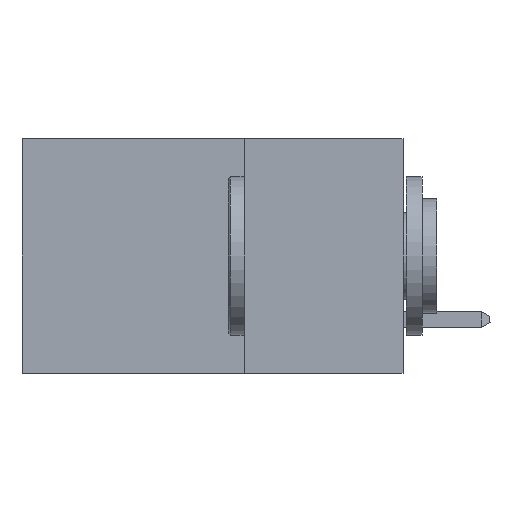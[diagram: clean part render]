
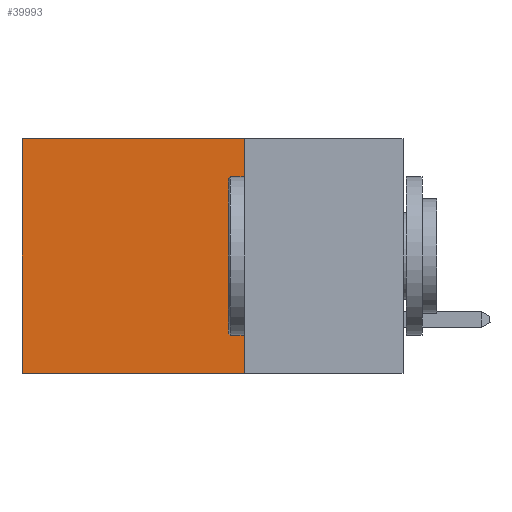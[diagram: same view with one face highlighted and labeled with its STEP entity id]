
A CAD part, left-side view. The second image highlights one B-rep face of the part: STEP entity #39993.
In plain terms, the highlighted planar face has unit normal (-1, 0, 0).
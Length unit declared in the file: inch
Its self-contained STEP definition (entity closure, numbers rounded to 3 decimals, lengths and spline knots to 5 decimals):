
#28 = EDGE_CURVE ( 'NONE', #30803, #10720, #9996, .T. ) ;
#980 = FACE_OUTER_BOUND ( 'NONE', #20535, .T. ) ;
#2550 = CARTESIAN_POINT ( 'NONE',  ( 0.2875, 0.25, 0. ) ) ;
#3827 = PLANE ( 'NONE',  #40299 ) ;
#6560 = DIRECTION ( 'NONE',  ( 0., 0., -1. ) ) ;
#7471 = ORIENTED_EDGE ( 'NONE', *, *, #28, .T. ) ;
#7860 = EDGE_CURVE ( 'NONE', #35607, #10720, #25566, .T. ) ;
#9996 = LINE ( 'NONE', #38169, #14913 ) ;
#10720 = VERTEX_POINT ( 'NONE', #34010 ) ;
#11876 = CARTESIAN_POINT ( 'NONE',  ( 0.2875, 0.25, 0. ) ) ;
#14913 = VECTOR ( 'NONE', #19667, 39.37008 ) ;
#15491 = VECTOR ( 'NONE', #36785, 39.37008 ) ;
#16440 = LINE ( 'NONE', #11876, #15491 ) ;
#17314 = VECTOR ( 'NONE', #28968, 39.37008 ) ;
#17499 = DIRECTION ( 'NONE',  ( 0., 1., 0. ) ) ;
#19667 = DIRECTION ( 'NONE',  ( 0., 0., -1. ) ) ;
#20377 = CARTESIAN_POINT ( 'NONE',  ( 0.2875, 0.25, 0. ) ) ;
#20535 = EDGE_LOOP ( 'NONE', ( #7471, #28157, #27523, #28884 ) ) ;
#23244 = CARTESIAN_POINT ( 'NONE',  ( 0.2875, 0.25, -0.37 ) ) ;
#25185 = CARTESIAN_POINT ( 'NONE',  ( 0.2875, 0.25, 0. ) ) ;
#25566 = LINE ( 'NONE', #23244, #17314 ) ;
#27523 = ORIENTED_EDGE ( 'NONE', *, *, #36398, .F. ) ;
#28067 = LINE ( 'NONE', #20377, #35387 ) ;
#28157 = ORIENTED_EDGE ( 'NONE', *, *, #7860, .F. ) ;
#28310 = EDGE_CURVE ( 'NONE', #33961, #30803, #28067, .T. ) ;
#28884 = ORIENTED_EDGE ( 'NONE', *, *, #28310, .T. ) ;
#28968 = DIRECTION ( 'NONE',  ( 0., 1., 0. ) ) ;
#30803 = VERTEX_POINT ( 'NONE', #34802 ) ;
#33961 = VERTEX_POINT ( 'NONE', #2550 ) ;
#34010 = CARTESIAN_POINT ( 'NONE',  ( 0.2875, 0.6, -0.37 ) ) ;
#34802 = CARTESIAN_POINT ( 'NONE',  ( 0.2875, 0.6, 0. ) ) ;
#35387 = VECTOR ( 'NONE', #17499, 39.37008 ) ;
#35607 = VERTEX_POINT ( 'NONE', #39144 ) ;
#36398 = EDGE_CURVE ( 'NONE', #33961, #35607, #16440, .T. ) ;
#36785 = DIRECTION ( 'NONE',  ( 0., 0., -1. ) ) ;
#37710 = DIRECTION ( 'NONE',  ( 1., 0., 0. ) ) ;
#38169 = CARTESIAN_POINT ( 'NONE',  ( 0.2875, 0.6, 0. ) ) ;
#39144 = CARTESIAN_POINT ( 'NONE',  ( 0.2875, 0.25, -0.37 ) ) ;
#39993 = ADVANCED_FACE ( 'NONE', ( #980 ), #3827, .F. ) ;
#40299 = AXIS2_PLACEMENT_3D ( 'NONE', #25185, #37710, #6560 ) ;
